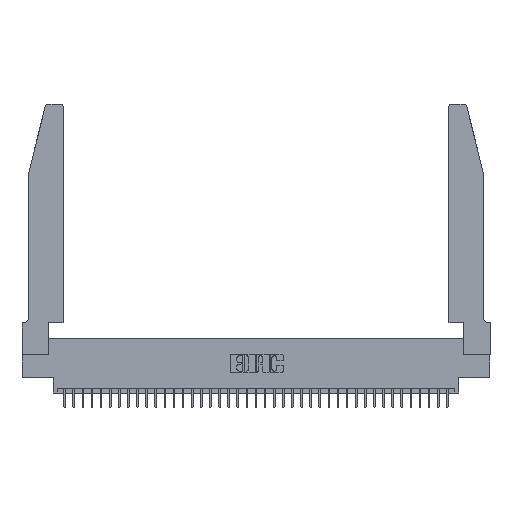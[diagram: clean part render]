
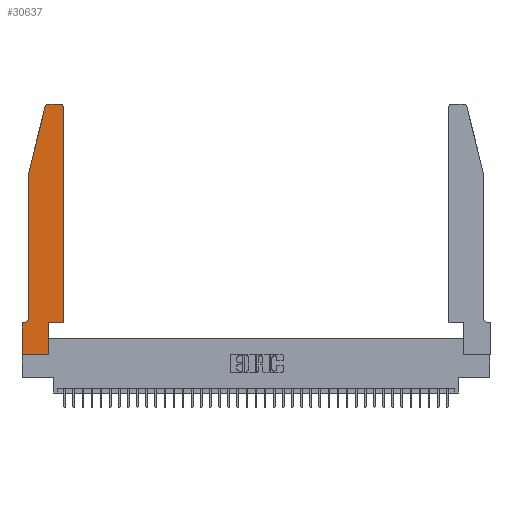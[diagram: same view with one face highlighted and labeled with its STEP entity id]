
A CAD part, top view. The second image highlights one B-rep face of the part: STEP entity #30637.
In plain terms, the highlighted planar face has unit normal (0, 0, 1).
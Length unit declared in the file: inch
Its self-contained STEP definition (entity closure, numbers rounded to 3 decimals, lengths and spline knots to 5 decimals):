
#288 = CARTESIAN_POINT ( 'NONE',  ( 0.0055, 0.42, 0.37 ) ) ;
#942 = AXIS2_PLACEMENT_3D ( 'NONE', #288, #21155, #3311 ) ;
#1195 = DIRECTION ( 'NONE',  ( 0., 1., 0. ) ) ;
#1209 = ORIENTED_EDGE ( 'NONE', *, *, #11223, .T. ) ;
#1630 = DIRECTION ( 'NONE',  ( 0., 1., 0. ) ) ;
#2388 = VERTEX_POINT ( 'NONE', #5349 ) ;
#2709 = DIRECTION ( 'NONE',  ( 0., 0., 1. ) ) ;
#2953 = CARTESIAN_POINT ( 'NONE',  ( 0.4505, 0.35, 0.37 ) ) ;
#3311 = DIRECTION ( 'NONE',  ( -1., 0., 0. ) ) ;
#4767 = PLANE ( 'NONE',  #8469 ) ;
#5349 = CARTESIAN_POINT ( 'NONE',  ( 0.2865, 0.35, 0.37 ) ) ;
#5754 = LINE ( 'NONE', #17364, #21545 ) ;
#5943 = CARTESIAN_POINT ( 'NONE',  ( 0.2865, 0., 0.37 ) ) ;
#6086 = VECTOR ( 'NONE', #12796, 39.37008 ) ;
#7838 = ORIENTED_EDGE ( 'NONE', *, *, #28182, .T. ) ;
#7934 = VERTEX_POINT ( 'NONE', #22530 ) ;
#8403 = VECTOR ( 'NONE', #1195, 39.37008 ) ;
#8469 = AXIS2_PLACEMENT_3D ( 'NONE', #28544, #10749, #31560 ) ;
#8541 = FACE_OUTER_BOUND ( 'NONE', #20235, .T. ) ;
#8749 = EDGE_CURVE ( 'NONE', #9088, #32179, #21452, .T. ) ;
#8852 = VECTOR ( 'NONE', #17015, 39.37008 ) ;
#9088 = VERTEX_POINT ( 'NONE', #34562 ) ;
#9460 = EDGE_CURVE ( 'NONE', #7934, #17103, #26990, .T. ) ;
#9678 = ORIENTED_EDGE ( 'NONE', *, *, #32540, .T. ) ;
#9727 = EDGE_CURVE ( 'NONE', #32179, #21858, #27035, .T. ) ;
#9757 = DIRECTION ( 'NONE',  ( 0., 0., 1. ) ) ;
#9818 = CARTESIAN_POINT ( 'NONE',  ( 0., 0., 0.37 ) ) ;
#10471 = CARTESIAN_POINT ( 'NONE',  ( 0., 0., 0.37 ) ) ;
#10618 = ORIENTED_EDGE ( 'NONE', *, *, #22958, .T. ) ;
#10749 = DIRECTION ( 'NONE',  ( 0., 0., 1. ) ) ;
#11216 = VECTOR ( 'NONE', #13762, 39.37008 ) ;
#11223 = EDGE_CURVE ( 'NONE', #33231, #25537, #36211, .T. ) ;
#12260 = LINE ( 'NONE', #10471, #29925 ) ;
#12796 = DIRECTION ( 'NONE',  ( 1., 0., 0. ) ) ;
#13043 = LINE ( 'NONE', #9818, #6086 ) ;
#13762 = DIRECTION ( 'NONE',  ( -1., 0., 0. ) ) ;
#13855 = ORIENTED_EDGE ( 'NONE', *, *, #9727, .T. ) ;
#14034 = CARTESIAN_POINT ( 'NONE',  ( 0.284, 2.75, 0.37 ) ) ;
#15763 = AXIS2_PLACEMENT_3D ( 'NONE', #20563, #2709, #23554 ) ;
#16087 = CARTESIAN_POINT ( 'NONE',  ( 0.2865, 0.35, 0.37 ) ) ;
#16740 = LINE ( 'NONE', #28815, #8852 ) ;
#16793 = LINE ( 'NONE', #37193, #31675 ) ;
#17015 = DIRECTION ( 'NONE',  ( -1., 0., 0. ) ) ;
#17103 = VERTEX_POINT ( 'NONE', #25163 ) ;
#17364 = CARTESIAN_POINT ( 'NONE',  ( 0.0755, 2., 0.37 ) ) ;
#17605 = ORIENTED_EDGE ( 'NONE', *, *, #18003, .T. ) ;
#18003 = EDGE_CURVE ( 'NONE', #2388, #23065, #38347, .T. ) ;
#18872 = CARTESIAN_POINT ( 'NONE',  ( 0.25487, 2.72718, 0.37 ) ) ;
#19526 = CARTESIAN_POINT ( 'NONE',  ( 0., 0., 0.37 ) ) ;
#20235 = EDGE_LOOP ( 'NONE', ( #24094, #1209, #25024, #34827, #36656, #13855, #29667, #7838, #9678, #17605, #10618, #20395 ) ) ;
#20395 = ORIENTED_EDGE ( 'NONE', *, *, #9460, .T. ) ;
#20563 = CARTESIAN_POINT ( 'NONE',  ( 0.284, 2.72, 0.37 ) ) ;
#20813 = DIRECTION ( 'NONE',  ( 1., 0., 0. ) ) ;
#21120 = DIRECTION ( 'NONE',  ( -0.239, -0.971, 0. ) ) ;
#21155 = DIRECTION ( 'NONE',  ( 0., 0., -1. ) ) ;
#21452 = CIRCLE ( 'NONE', #942, 0.07 ) ;
#21466 = AXIS2_PLACEMENT_3D ( 'NONE', #27570, #9757, #30519 ) ;
#21545 = VECTOR ( 'NONE', #38163, 39.37008 ) ;
#21858 = VERTEX_POINT ( 'NONE', #26111 ) ;
#22522 = VECTOR ( 'NONE', #20813, 39.37008 ) ;
#22530 = CARTESIAN_POINT ( 'NONE',  ( 0.4505, 2.72, 0.37 ) ) ;
#22958 = EDGE_CURVE ( 'NONE', #23065, #7934, #16793, .T. ) ;
#23065 = VERTEX_POINT ( 'NONE', #37830 ) ;
#23554 = DIRECTION ( 'NONE',  ( 1., 0., 0. ) ) ;
#23596 = LINE ( 'NONE', #29937, #30520 ) ;
#24094 = ORIENTED_EDGE ( 'NONE', *, *, #32719, .T. ) ;
#24201 = LINE ( 'NONE', #16087, #8403 ) ;
#24336 = VERTEX_POINT ( 'NONE', #31372 ) ;
#25024 = ORIENTED_EDGE ( 'NONE', *, *, #28403, .T. ) ;
#25163 = CARTESIAN_POINT ( 'NONE',  ( 0.4205, 2.75, 0.37 ) ) ;
#25537 = VERTEX_POINT ( 'NONE', #18872 ) ;
#26111 = CARTESIAN_POINT ( 'NONE',  ( 0., 0.35, 0.37 ) ) ;
#26534 = CARTESIAN_POINT ( 'NONE',  ( 0.0055, 0.35, 0.37 ) ) ;
#26990 = CIRCLE ( 'NONE', #21466, 0.03 ) ;
#27035 = LINE ( 'NONE', #34614, #11216 ) ;
#27570 = CARTESIAN_POINT ( 'NONE',  ( 0.4205, 2.72, 0.37 ) ) ;
#28182 = EDGE_CURVE ( 'NONE', #37444, #32903, #13043, .T. ) ;
#28273 = DIRECTION ( 'NONE',  ( 0., -1., 0. ) ) ;
#28403 = EDGE_CURVE ( 'NONE', #25537, #24336, #23596, .T. ) ;
#28544 = CARTESIAN_POINT ( 'NONE',  ( 0., 0.35, 0.37 ) ) ;
#28815 = CARTESIAN_POINT ( 'NONE',  ( 0.2605, 2.75, 0.37 ) ) ;
#29667 = ORIENTED_EDGE ( 'NONE', *, *, #36776, .T. ) ;
#29925 = VECTOR ( 'NONE', #28273, 39.37008 ) ;
#29937 = CARTESIAN_POINT ( 'NONE',  ( 0.0755, 2., 0.37 ) ) ;
#30519 = DIRECTION ( 'NONE',  ( 1., 0., 0. ) ) ;
#30520 = VECTOR ( 'NONE', #21120, 39.37008 ) ;
#30637 = ADVANCED_FACE ( 'NONE', ( #8541 ), #4767, .T. ) ;
#31372 = CARTESIAN_POINT ( 'NONE',  ( 0.0755, 2., 0.37 ) ) ;
#31560 = DIRECTION ( 'NONE',  ( 1., 0., 0. ) ) ;
#31675 = VECTOR ( 'NONE', #1630, 39.37008 ) ;
#32179 = VERTEX_POINT ( 'NONE', #26534 ) ;
#32540 = EDGE_CURVE ( 'NONE', #32903, #2388, #24201, .T. ) ;
#32719 = EDGE_CURVE ( 'NONE', #17103, #33231, #16740, .T. ) ;
#32903 = VERTEX_POINT ( 'NONE', #5943 ) ;
#33231 = VERTEX_POINT ( 'NONE', #14034 ) ;
#34562 = CARTESIAN_POINT ( 'NONE',  ( 0.0755, 0.42, 0.37 ) ) ;
#34614 = CARTESIAN_POINT ( 'NONE',  ( 0.0755, 0.35, 0.37 ) ) ;
#34827 = ORIENTED_EDGE ( 'NONE', *, *, #36950, .T. ) ;
#36211 = CIRCLE ( 'NONE', #15763, 0.03 ) ;
#36656 = ORIENTED_EDGE ( 'NONE', *, *, #8749, .T. ) ;
#36776 = EDGE_CURVE ( 'NONE', #21858, #37444, #12260, .T. ) ;
#36950 = EDGE_CURVE ( 'NONE', #24336, #9088, #5754, .T. ) ;
#37193 = CARTESIAN_POINT ( 'NONE',  ( 0.4505, 0.35, 0.37 ) ) ;
#37444 = VERTEX_POINT ( 'NONE', #19526 ) ;
#37830 = CARTESIAN_POINT ( 'NONE',  ( 0.4505, 0.35, 0.37 ) ) ;
#38163 = DIRECTION ( 'NONE',  ( 0., -1., 0. ) ) ;
#38347 = LINE ( 'NONE', #2953, #22522 ) ;
